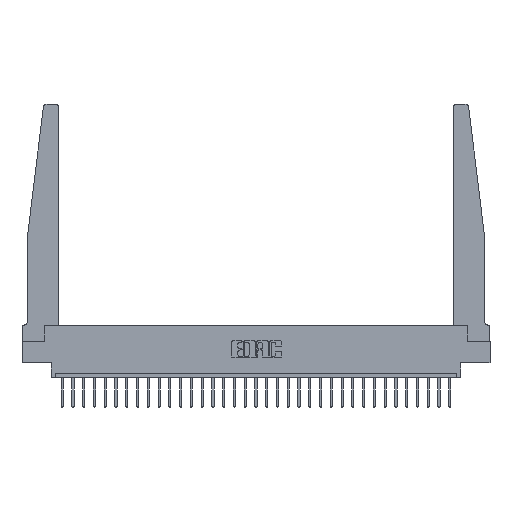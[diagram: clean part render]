
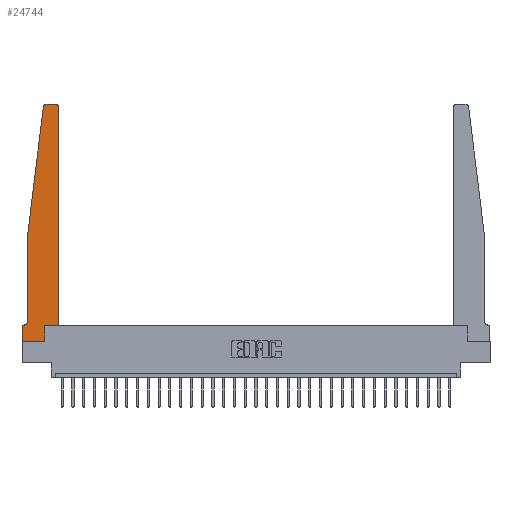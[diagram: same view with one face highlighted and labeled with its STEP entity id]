
A CAD part, top view. The second image highlights one B-rep face of the part: STEP entity #24744.
In plain terms, the highlighted planar face has unit normal (0, 0, 1).
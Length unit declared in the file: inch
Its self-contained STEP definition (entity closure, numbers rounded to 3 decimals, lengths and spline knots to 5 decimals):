
#76 = EDGE_CURVE ( 'NONE', #7772, #21560, #4694, .T. ) ;
#568 = EDGE_CURVE ( 'NONE', #5569, #12524, #9135, .T. ) ;
#804 = DIRECTION ( 'NONE',  ( 0., 0., -1. ) ) ;
#891 = CIRCLE ( 'NONE', #9836, 0.03 ) ;
#1267 = VECTOR ( 'NONE', #23355, 39.37008 ) ;
#1909 = AXIS2_PLACEMENT_3D ( 'NONE', #27201, #804, #16180 ) ;
#2636 = CARTESIAN_POINT ( 'NONE',  ( 0.2605, 0.18, 0.37 ) ) ;
#3592 = CARTESIAN_POINT ( 'NONE',  ( 0.2605, 0.18, 0.37 ) ) ;
#3714 = CARTESIAN_POINT ( 'NONE',  ( 0.425, 0.18, 0.37 ) ) ;
#4400 = LINE ( 'NONE', #19292, #9570 ) ;
#4694 = LINE ( 'NONE', #5788, #1267 ) ;
#4699 = VERTEX_POINT ( 'NONE', #18985 ) ;
#4974 = CIRCLE ( 'NONE', #1909, 0.05 ) ;
#5000 = DIRECTION ( 'NONE',  ( -1., 0., 0. ) ) ;
#5296 = EDGE_CURVE ( 'NONE', #4699, #18547, #20815, .T. ) ;
#5353 = ORIENTED_EDGE ( 'NONE', *, *, #18929, .T. ) ;
#5452 = VECTOR ( 'NONE', #10103, 39.37008 ) ;
#5569 = VERTEX_POINT ( 'NONE', #25542 ) ;
#5788 = CARTESIAN_POINT ( 'NONE',  ( 0.065, 1.25, 0.37 ) ) ;
#5886 = CARTESIAN_POINT ( 'NONE',  ( 0.425, 0.18, 0.37 ) ) ;
#5940 = VERTEX_POINT ( 'NONE', #5886 ) ;
#6519 = ORIENTED_EDGE ( 'NONE', *, *, #14328, .T. ) ;
#7148 = LINE ( 'NONE', #25396, #24100 ) ;
#7429 = EDGE_LOOP ( 'NONE', ( #15403, #16224, #6519, #17728, #5353, #22578, #11447, #10684, #15721, #26131, #9033, #22200 ) ) ;
#7772 = VERTEX_POINT ( 'NONE', #20535 ) ;
#7914 = EDGE_CURVE ( 'NONE', #20192, #4699, #15516, .T. ) ;
#8509 = VERTEX_POINT ( 'NONE', #10371 ) ;
#9033 = ORIENTED_EDGE ( 'NONE', *, *, #10037, .T. ) ;
#9135 = LINE ( 'NONE', #22649, #26070 ) ;
#9327 = DIRECTION ( 'NONE',  ( 0., 0., 1. ) ) ;
#9570 = VECTOR ( 'NONE', #21322, 39.37008 ) ;
#9836 = AXIS2_PLACEMENT_3D ( 'NONE', #22522, #9327, #13762 ) ;
#10037 = EDGE_CURVE ( 'NONE', #5940, #28549, #21077, .T. ) ;
#10103 = DIRECTION ( 'NONE',  ( -1., 0., 0. ) ) ;
#10371 = CARTESIAN_POINT ( 'NONE',  ( 0.27653, 2.75, 0.37 ) ) ;
#10684 = ORIENTED_EDGE ( 'NONE', *, *, #7914, .T. ) ;
#11447 = ORIENTED_EDGE ( 'NONE', *, *, #15589, .T. ) ;
#11975 = VERTEX_POINT ( 'NONE', #16408 ) ;
#12422 = CARTESIAN_POINT ( 'NONE',  ( 0.395, 2.72, 0.37 ) ) ;
#12524 = VERTEX_POINT ( 'NONE', #14354 ) ;
#13762 = DIRECTION ( 'NONE',  ( 1., 0., 0. ) ) ;
#13770 = VECTOR ( 'NONE', #17739, 39.37008 ) ;
#14328 = EDGE_CURVE ( 'NONE', #25043, #7772, #17578, .T. ) ;
#14354 = CARTESIAN_POINT ( 'NONE',  ( 0., 0.1875, 0.37 ) ) ;
#14933 = EDGE_CURVE ( 'NONE', #18547, #5940, #7148, .T. ) ;
#15403 = ORIENTED_EDGE ( 'NONE', *, *, #22592, .T. ) ;
#15516 = LINE ( 'NONE', #26523, #20003 ) ;
#15589 = EDGE_CURVE ( 'NONE', #12524, #20192, #4400, .T. ) ;
#15721 = ORIENTED_EDGE ( 'NONE', *, *, #5296, .T. ) ;
#16180 = DIRECTION ( 'NONE',  ( -1., 0., 0. ) ) ;
#16224 = ORIENTED_EDGE ( 'NONE', *, *, #25751, .T. ) ;
#16408 = CARTESIAN_POINT ( 'NONE',  ( 0.395, 2.75, 0.37 ) ) ;
#16697 = VECTOR ( 'NONE', #24494, 39.37008 ) ;
#16955 = DIRECTION ( 'NONE',  ( 0., 0., 1. ) ) ;
#17011 = DIRECTION ( 'NONE',  ( 0., 1., 0. ) ) ;
#17021 = PLANE ( 'NONE',  #26811 ) ;
#17578 = LINE ( 'NONE', #24095, #13770 ) ;
#17728 = ORIENTED_EDGE ( 'NONE', *, *, #76, .T. ) ;
#17739 = DIRECTION ( 'NONE',  ( -0.122, -0.992, 0. ) ) ;
#18547 = VERTEX_POINT ( 'NONE', #3592 ) ;
#18794 = CARTESIAN_POINT ( 'NONE',  ( 0.065, 0.2375, 0.37 ) ) ;
#18830 = DIRECTION ( 'NONE',  ( 1., 0., 0. ) ) ;
#18929 = EDGE_CURVE ( 'NONE', #21560, #5569, #4974, .T. ) ;
#18985 = CARTESIAN_POINT ( 'NONE',  ( 0.2605, 0., 0.37 ) ) ;
#19292 = CARTESIAN_POINT ( 'NONE',  ( 0., 0., 0.37 ) ) ;
#20003 = VECTOR ( 'NONE', #26705, 39.37008 ) ;
#20192 = VERTEX_POINT ( 'NONE', #23356 ) ;
#20535 = CARTESIAN_POINT ( 'NONE',  ( 0.065, 1.25, 0.37 ) ) ;
#20815 = LINE ( 'NONE', #2636, #16697 ) ;
#21077 = LINE ( 'NONE', #3714, #27289 ) ;
#21274 = DIRECTION ( 'NONE',  ( 1., 0., 0. ) ) ;
#21322 = DIRECTION ( 'NONE',  ( 0., -1., 0. ) ) ;
#21336 = DIRECTION ( 'NONE',  ( 0., 0., 1. ) ) ;
#21560 = VERTEX_POINT ( 'NONE', #18794 ) ;
#21808 = AXIS2_PLACEMENT_3D ( 'NONE', #12422, #16955, #21274 ) ;
#22200 = ORIENTED_EDGE ( 'NONE', *, *, #24105, .T. ) ;
#22522 = CARTESIAN_POINT ( 'NONE',  ( 0.27653, 2.72, 0.37 ) ) ;
#22578 = ORIENTED_EDGE ( 'NONE', *, *, #568, .T. ) ;
#22592 = EDGE_CURVE ( 'NONE', #11975, #8509, #24768, .T. ) ;
#22649 = CARTESIAN_POINT ( 'NONE',  ( 0.065, 0.1875, 0.37 ) ) ;
#23297 = CARTESIAN_POINT ( 'NONE',  ( 0.25, 2.75, 0.37 ) ) ;
#23355 = DIRECTION ( 'NONE',  ( 0., -1., 0. ) ) ;
#23356 = CARTESIAN_POINT ( 'NONE',  ( 0., 0., 0.37 ) ) ;
#24050 = FACE_OUTER_BOUND ( 'NONE', #7429, .T. ) ;
#24095 = CARTESIAN_POINT ( 'NONE',  ( 0.065, 1.25, 0.37 ) ) ;
#24100 = VECTOR ( 'NONE', #18830, 39.37008 ) ;
#24105 = EDGE_CURVE ( 'NONE', #28549, #11975, #25425, .T. ) ;
#24494 = DIRECTION ( 'NONE',  ( 0., 1., 0. ) ) ;
#24744 = ADVANCED_FACE ( 'NONE', ( #24050 ), #17021, .T. ) ;
#24768 = LINE ( 'NONE', #23297, #5452 ) ;
#25043 = VERTEX_POINT ( 'NONE', #26901 ) ;
#25396 = CARTESIAN_POINT ( 'NONE',  ( 0.425, 0.18, 0.37 ) ) ;
#25425 = CIRCLE ( 'NONE', #21808, 0.03 ) ;
#25542 = CARTESIAN_POINT ( 'NONE',  ( 0.015, 0.1875, 0.37 ) ) ;
#25685 = CARTESIAN_POINT ( 'NONE',  ( 0., 0.1875, 0.37 ) ) ;
#25751 = EDGE_CURVE ( 'NONE', #8509, #25043, #891, .T. ) ;
#25880 = DIRECTION ( 'NONE',  ( 1., 0., 0. ) ) ;
#26070 = VECTOR ( 'NONE', #5000, 39.37008 ) ;
#26131 = ORIENTED_EDGE ( 'NONE', *, *, #14933, .T. ) ;
#26523 = CARTESIAN_POINT ( 'NONE',  ( 0., 0., 0.37 ) ) ;
#26705 = DIRECTION ( 'NONE',  ( 1., 0., 0. ) ) ;
#26811 = AXIS2_PLACEMENT_3D ( 'NONE', #25685, #21336, #25880 ) ;
#26901 = CARTESIAN_POINT ( 'NONE',  ( 0.24675, 2.72367, 0.37 ) ) ;
#27156 = CARTESIAN_POINT ( 'NONE',  ( 0.425, 2.72, 0.37 ) ) ;
#27201 = CARTESIAN_POINT ( 'NONE',  ( 0.015, 0.2375, 0.37 ) ) ;
#27289 = VECTOR ( 'NONE', #17011, 39.37008 ) ;
#28549 = VERTEX_POINT ( 'NONE', #27156 ) ;
